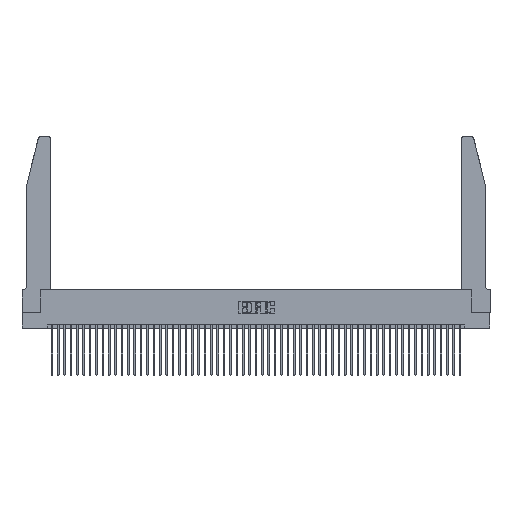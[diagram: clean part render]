
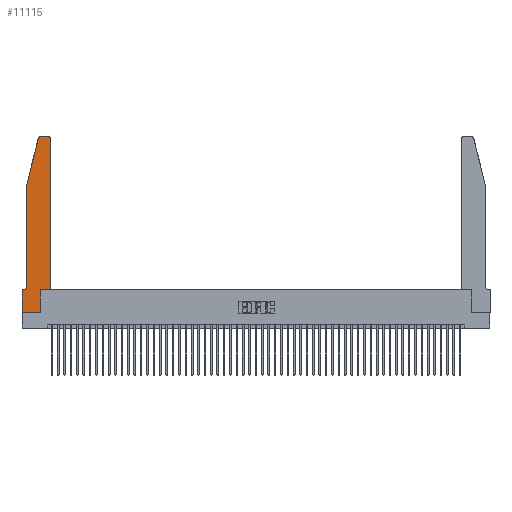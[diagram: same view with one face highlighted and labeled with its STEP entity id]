
A CAD part, top view. The second image highlights one B-rep face of the part: STEP entity #11115.
In plain terms, the highlighted planar face has unit normal (0, 0, 1).
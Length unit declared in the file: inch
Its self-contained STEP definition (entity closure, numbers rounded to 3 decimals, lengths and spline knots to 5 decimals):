
#768 = CARTESIAN_POINT ( 'NONE',  ( 0., 0., 0.37 ) ) ;
#1737 = CIRCLE ( 'NONE', #14310, 0.03 ) ;
#1947 = VERTEX_POINT ( 'NONE', #23293 ) ;
#2497 = ORIENTED_EDGE ( 'NONE', *, *, #26332, .T. ) ;
#4145 = VERTEX_POINT ( 'NONE', #40106 ) ;
#4573 = DIRECTION ( 'NONE',  ( 0., 0., 1. ) ) ;
#5269 = VERTEX_POINT ( 'NONE', #36596 ) ;
#5379 = VECTOR ( 'NONE', #48546, 39.37008 ) ;
#5991 = VECTOR ( 'NONE', #22834, 39.37008 ) ;
#6755 = ORIENTED_EDGE ( 'NONE', *, *, #45583, .T. ) ;
#7931 = CARTESIAN_POINT ( 'NONE',  ( 0., 0.35, 0.37 ) ) ;
#8687 = ORIENTED_EDGE ( 'NONE', *, *, #17893, .T. ) ;
#11115 = ADVANCED_FACE ( 'NONE', ( #23939 ), #38455, .T. ) ;
#11871 = ORIENTED_EDGE ( 'NONE', *, *, #16962, .T. ) ;
#12947 = EDGE_CURVE ( 'NONE', #47734, #42228, #1737, .T. ) ;
#13500 = DIRECTION ( 'NONE',  ( 0., 0., 1. ) ) ;
#13716 = EDGE_CURVE ( 'NONE', #1947, #21402, #50796, .T. ) ;
#14310 = AXIS2_PLACEMENT_3D ( 'NONE', #37754, #13500, #41754 ) ;
#14520 = EDGE_CURVE ( 'NONE', #42977, #1947, #43795, .T. ) ;
#15195 = CIRCLE ( 'NONE', #36798, 0.07 ) ;
#16962 = EDGE_CURVE ( 'NONE', #21402, #36624, #15195, .T. ) ;
#17183 = CARTESIAN_POINT ( 'NONE',  ( 0.4505, 2.72, 0.37 ) ) ;
#17195 = EDGE_LOOP ( 'NONE', ( #6755, #40708, #39786, #36868, #11871, #8687, #34847, #33595, #44623, #2497, #52605, #24248 ) ) ;
#17211 = VERTEX_POINT ( 'NONE', #48782 ) ;
#17893 = EDGE_CURVE ( 'NONE', #36624, #46957, #37878, .T. ) ;
#18170 = CARTESIAN_POINT ( 'NONE',  ( 0., 0.35, 0.37 ) ) ;
#18351 = DIRECTION ( 'NONE',  ( 1., 0., 0. ) ) ;
#18697 = AXIS2_PLACEMENT_3D ( 'NONE', #18170, #42464, #18351 ) ;
#18700 = CARTESIAN_POINT ( 'NONE',  ( 0.2605, 2.75, 0.37 ) ) ;
#18825 = CARTESIAN_POINT ( 'NONE',  ( 0.0755, 2., 0.37 ) ) ;
#18888 = CARTESIAN_POINT ( 'NONE',  ( 0.0055, 0.42, 0.37 ) ) ;
#18898 = CARTESIAN_POINT ( 'NONE',  ( 0.25487, 2.72718, 0.37 ) ) ;
#18899 = LINE ( 'NONE', #42843, #27178 ) ;
#19580 = DIRECTION ( 'NONE',  ( 0., 1., 0. ) ) ;
#21346 = VECTOR ( 'NONE', #46351, 39.37008 ) ;
#21402 = VERTEX_POINT ( 'NONE', #23068 ) ;
#22400 = CARTESIAN_POINT ( 'NONE',  ( 0.4205, 2.75, 0.37 ) ) ;
#22834 = DIRECTION ( 'NONE',  ( -1., 0., 0. ) ) ;
#23031 = DIRECTION ( 'NONE',  ( -1., 0., 0. ) ) ;
#23068 = CARTESIAN_POINT ( 'NONE',  ( 0.0755, 0.42, 0.37 ) ) ;
#23293 = CARTESIAN_POINT ( 'NONE',  ( 0.0755, 2., 0.37 ) ) ;
#23939 = FACE_OUTER_BOUND ( 'NONE', #17195, .T. ) ;
#24248 = ORIENTED_EDGE ( 'NONE', *, *, #12947, .T. ) ;
#26059 = DIRECTION ( 'NONE',  ( 1., 0., 0. ) ) ;
#26332 = EDGE_CURVE ( 'NONE', #4145, #5269, #38289, .T. ) ;
#27178 = VECTOR ( 'NONE', #38997, 39.37008 ) ;
#28896 = VECTOR ( 'NONE', #26059, 39.37008 ) ;
#29057 = LINE ( 'NONE', #18700, #5991 ) ;
#29154 = CARTESIAN_POINT ( 'NONE',  ( 0.284, 2.72, 0.37 ) ) ;
#29442 = CIRCLE ( 'NONE', #34355, 0.03 ) ;
#32048 = VECTOR ( 'NONE', #41616, 39.37008 ) ;
#33196 = DIRECTION ( 'NONE',  ( 1., 0., 0. ) ) ;
#33225 = CARTESIAN_POINT ( 'NONE',  ( 0., 0., 0.37 ) ) ;
#33338 = CARTESIAN_POINT ( 'NONE',  ( 0.2865, 0., 0.37 ) ) ;
#33350 = LINE ( 'NONE', #50244, #21346 ) ;
#33595 = ORIENTED_EDGE ( 'NONE', *, *, #34939, .T. ) ;
#34355 = AXIS2_PLACEMENT_3D ( 'NONE', #29154, #4573, #33196 ) ;
#34847 = ORIENTED_EDGE ( 'NONE', *, *, #36626, .T. ) ;
#34939 = EDGE_CURVE ( 'NONE', #51117, #49846, #18899, .T. ) ;
#34998 = LINE ( 'NONE', #43682, #45644 ) ;
#36596 = CARTESIAN_POINT ( 'NONE',  ( 0.4505, 0.35, 0.37 ) ) ;
#36624 = VERTEX_POINT ( 'NONE', #45493 ) ;
#36626 = EDGE_CURVE ( 'NONE', #46957, #51117, #41385, .T. ) ;
#36798 = AXIS2_PLACEMENT_3D ( 'NONE', #18888, #47048, #23031 ) ;
#36868 = ORIENTED_EDGE ( 'NONE', *, *, #13716, .T. ) ;
#37162 = EDGE_CURVE ( 'NONE', #17211, #42977, #29442, .T. ) ;
#37754 = CARTESIAN_POINT ( 'NONE',  ( 0.4205, 2.72, 0.37 ) ) ;
#37878 = LINE ( 'NONE', #40466, #5379 ) ;
#38289 = LINE ( 'NONE', #50098, #28896 ) ;
#38455 = PLANE ( 'NONE',  #18697 ) ;
#38853 = VECTOR ( 'NONE', #46981, 39.37008 ) ;
#38997 = DIRECTION ( 'NONE',  ( 1., 0., 0. ) ) ;
#39786 = ORIENTED_EDGE ( 'NONE', *, *, #14520, .T. ) ;
#40106 = CARTESIAN_POINT ( 'NONE',  ( 0.2865, 0.35, 0.37 ) ) ;
#40466 = CARTESIAN_POINT ( 'NONE',  ( 0.0755, 0.35, 0.37 ) ) ;
#40708 = ORIENTED_EDGE ( 'NONE', *, *, #37162, .T. ) ;
#41385 = LINE ( 'NONE', #768, #32048 ) ;
#41616 = DIRECTION ( 'NONE',  ( 0., -1., 0. ) ) ;
#41754 = DIRECTION ( 'NONE',  ( 1., 0., 0. ) ) ;
#42228 = VERTEX_POINT ( 'NONE', #22400 ) ;
#42464 = DIRECTION ( 'NONE',  ( 0., 0., 1. ) ) ;
#42517 = VECTOR ( 'NONE', #44109, 39.37008 ) ;
#42843 = CARTESIAN_POINT ( 'NONE',  ( 0., 0., 0.37 ) ) ;
#42977 = VERTEX_POINT ( 'NONE', #18898 ) ;
#43682 = CARTESIAN_POINT ( 'NONE',  ( 0.4505, 0.35, 0.37 ) ) ;
#43795 = LINE ( 'NONE', #52178, #42517 ) ;
#44109 = DIRECTION ( 'NONE',  ( -0.239, -0.971, 0. ) ) ;
#44623 = ORIENTED_EDGE ( 'NONE', *, *, #46600, .T. ) ;
#45493 = CARTESIAN_POINT ( 'NONE',  ( 0.0055, 0.35, 0.37 ) ) ;
#45583 = EDGE_CURVE ( 'NONE', #42228, #17211, #29057, .T. ) ;
#45644 = VECTOR ( 'NONE', #19580, 39.37008 ) ;
#46351 = DIRECTION ( 'NONE',  ( 0., 1., 0. ) ) ;
#46600 = EDGE_CURVE ( 'NONE', #49846, #4145, #33350, .T. ) ;
#46957 = VERTEX_POINT ( 'NONE', #7931 ) ;
#46981 = DIRECTION ( 'NONE',  ( 0., -1., 0. ) ) ;
#47048 = DIRECTION ( 'NONE',  ( 0., 0., -1. ) ) ;
#47734 = VERTEX_POINT ( 'NONE', #17183 ) ;
#48546 = DIRECTION ( 'NONE',  ( -1., 0., 0. ) ) ;
#48782 = CARTESIAN_POINT ( 'NONE',  ( 0.284, 2.75, 0.37 ) ) ;
#49846 = VERTEX_POINT ( 'NONE', #33338 ) ;
#50098 = CARTESIAN_POINT ( 'NONE',  ( 0.4505, 0.35, 0.37 ) ) ;
#50244 = CARTESIAN_POINT ( 'NONE',  ( 0.2865, 0.35, 0.37 ) ) ;
#50796 = LINE ( 'NONE', #18825, #38853 ) ;
#51117 = VERTEX_POINT ( 'NONE', #33225 ) ;
#52178 = CARTESIAN_POINT ( 'NONE',  ( 0.0755, 2., 0.37 ) ) ;
#52272 = EDGE_CURVE ( 'NONE', #5269, #47734, #34998, .T. ) ;
#52605 = ORIENTED_EDGE ( 'NONE', *, *, #52272, .T. ) ;
